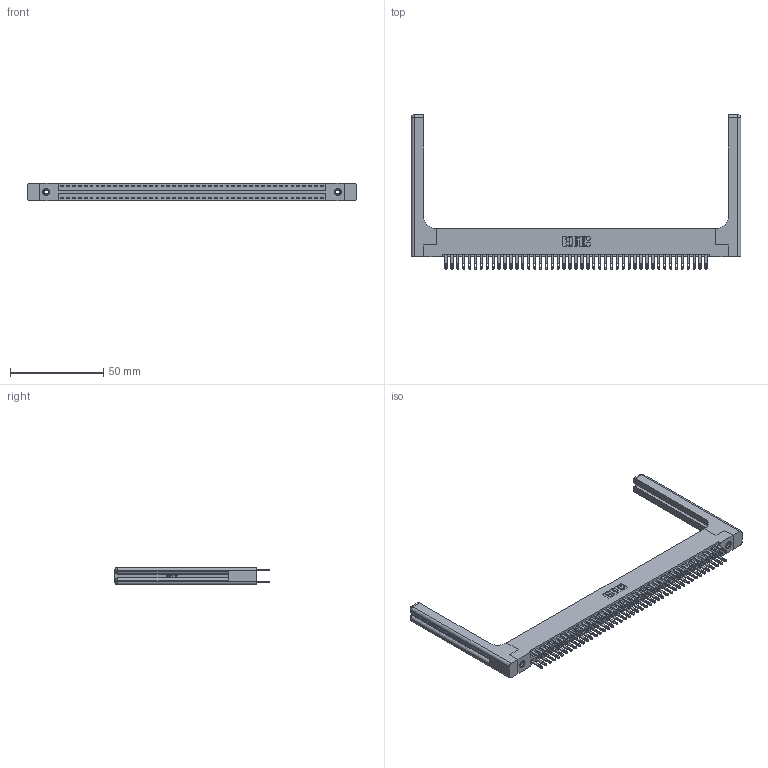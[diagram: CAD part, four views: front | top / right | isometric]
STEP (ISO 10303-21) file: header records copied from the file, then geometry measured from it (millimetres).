
FILE_DESCRIPTION (( 'STEP AP203' ), '1' );
FILE_NAME ('346-090-500-258.STEP', '2022-05-26T02:51:01', ( '' ), ( '' ), 'SwSTEP 2.0', 'SolidWorks 2020', '' );
FILE_SCHEMA (( 'CONFIG_CONTROL_DESIGN' ));
Length unit declared in the file: inch
Products named in the file (5): 346-220-058_345-220-058; 345-292-001_345-293-100; 346-090-500-258; 345-250-001_345-250-001-102; 346 Part_Flush Mounting Lugs - 0.156 Dia-TH
Assembly tree (95 placements, depth 2):
  346-090-500-258
    346 Part_Flush Mounting Lugs - 0.156 Dia-TH
    345-292-001_345-293-100  x90
    345-250-001_345-250-001-102  x2
    346-220-058_345-220-058  x2
Bounding box: 176.94 x 82.8 x 9.4 mm (x, y, z)
Volume: 25028 mm3; surface area: 30097.7 mm2
Topology: 95 solids, 95 shells, 4712 faces, 14261 edges, 9486 vertices
Faces by surface type: plane 2848, cylinder 1804, bspline 36, cone 12, sphere 8, torus 4
Entity records: 34492 total; most frequent: CARTESIAN_POINT 6691, ORIENTED_EDGE 5420, DIRECTION 4882, EDGE_CURVE 2710, VECTOR 2302, LINE 2302, VERTEX_POINT 1798, AXIS2_PLACEMENT_3D 1290
